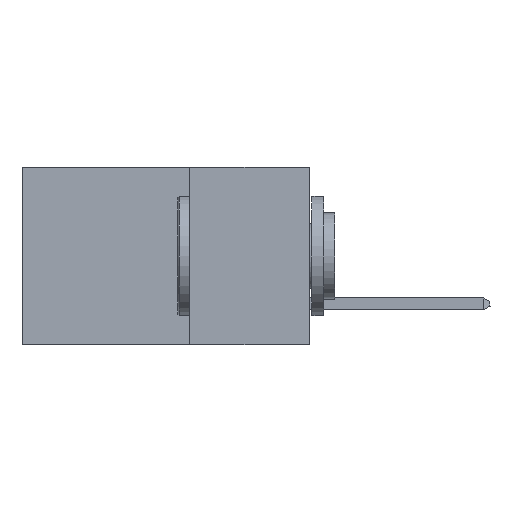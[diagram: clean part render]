
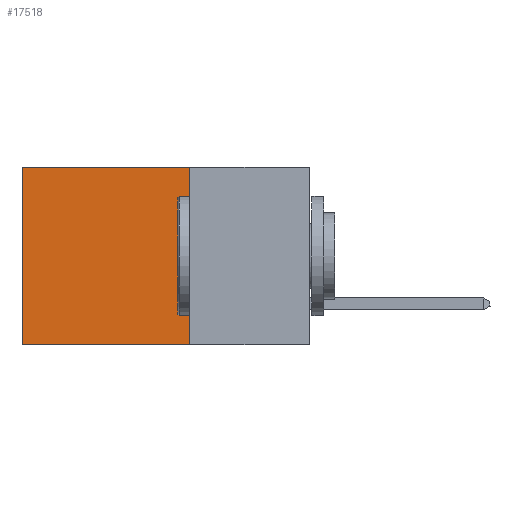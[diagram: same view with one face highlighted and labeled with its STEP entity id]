
A CAD part, left-side view. The second image highlights one B-rep face of the part: STEP entity #17518.
In plain terms, the highlighted planar face has unit normal (-1, 0, 0).
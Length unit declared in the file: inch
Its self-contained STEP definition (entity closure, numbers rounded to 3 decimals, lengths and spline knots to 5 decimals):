
#273 = VECTOR ( 'NONE', #21342, 39.37008 ) ;
#858 = ORIENTED_EDGE ( 'NONE', *, *, #24245, .F. ) ;
#1565 = LINE ( 'NONE', #18828, #15448 ) ;
#2583 = CARTESIAN_POINT ( 'NONE',  ( 0.2875, 0.6, 0. ) ) ;
#2757 = CARTESIAN_POINT ( 'NONE',  ( 0.2875, 0.25, -0.37 ) ) ;
#3006 = DIRECTION ( 'NONE',  ( 1., 0., 0. ) ) ;
#3164 = DIRECTION ( 'NONE',  ( 0., 1., 0. ) ) ;
#3931 = VECTOR ( 'NONE', #3164, 39.37008 ) ;
#4795 = LINE ( 'NONE', #19295, #273 ) ;
#5175 = CARTESIAN_POINT ( 'NONE',  ( 0.2875, 0.25, 0. ) ) ;
#5219 = LINE ( 'NONE', #14986, #3931 ) ;
#6112 = VERTEX_POINT ( 'NONE', #2757 ) ;
#6559 = PLANE ( 'NONE',  #7808 ) ;
#6691 = VERTEX_POINT ( 'NONE', #22443 ) ;
#6726 = FACE_OUTER_BOUND ( 'NONE', #12851, .T. ) ;
#7319 = CARTESIAN_POINT ( 'NONE',  ( 0.2875, 0.6, 0. ) ) ;
#7808 = AXIS2_PLACEMENT_3D ( 'NONE', #5175, #3006, #26166 ) ;
#9310 = DIRECTION ( 'NONE',  ( 0., 0., -1. ) ) ;
#10297 = EDGE_CURVE ( 'NONE', #18329, #6691, #22683, .T. ) ;
#12673 = ORIENTED_EDGE ( 'NONE', *, *, #14726, .T. ) ;
#12851 = EDGE_LOOP ( 'NONE', ( #12966, #858, #19882, #12673 ) ) ;
#12966 = ORIENTED_EDGE ( 'NONE', *, *, #10297, .T. ) ;
#14212 = CARTESIAN_POINT ( 'NONE',  ( 0.2875, 0.25, 0. ) ) ;
#14726 = EDGE_CURVE ( 'NONE', #23442, #18329, #5219, .T. ) ;
#14986 = CARTESIAN_POINT ( 'NONE',  ( 0.2875, 0.25, 0. ) ) ;
#15448 = VECTOR ( 'NONE', #25141, 39.37008 ) ;
#17131 = EDGE_CURVE ( 'NONE', #23442, #6112, #1565, .T. ) ;
#17518 = ADVANCED_FACE ( 'NONE', ( #6726 ), #6559, .F. ) ;
#18329 = VERTEX_POINT ( 'NONE', #2583 ) ;
#18828 = CARTESIAN_POINT ( 'NONE',  ( 0.2875, 0.25, 0. ) ) ;
#19295 = CARTESIAN_POINT ( 'NONE',  ( 0.2875, 0.25, -0.37 ) ) ;
#19882 = ORIENTED_EDGE ( 'NONE', *, *, #17131, .F. ) ;
#21342 = DIRECTION ( 'NONE',  ( 0., 1., 0. ) ) ;
#22443 = CARTESIAN_POINT ( 'NONE',  ( 0.2875, 0.6, -0.37 ) ) ;
#22683 = LINE ( 'NONE', #7319, #26592 ) ;
#23442 = VERTEX_POINT ( 'NONE', #14212 ) ;
#24245 = EDGE_CURVE ( 'NONE', #6112, #6691, #4795, .T. ) ;
#25141 = DIRECTION ( 'NONE',  ( 0., 0., -1. ) ) ;
#26166 = DIRECTION ( 'NONE',  ( 0., 0., -1. ) ) ;
#26592 = VECTOR ( 'NONE', #9310, 39.37008 ) ;
